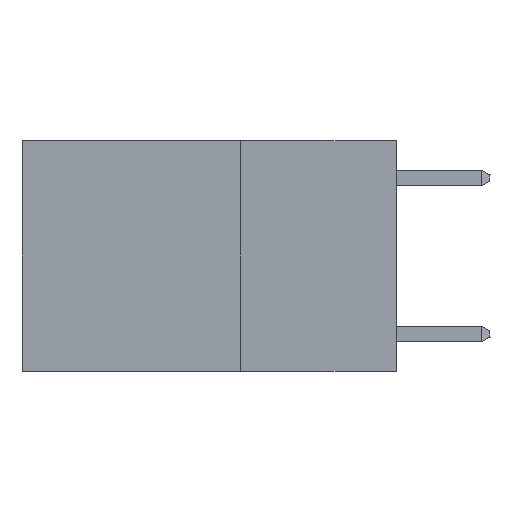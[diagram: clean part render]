
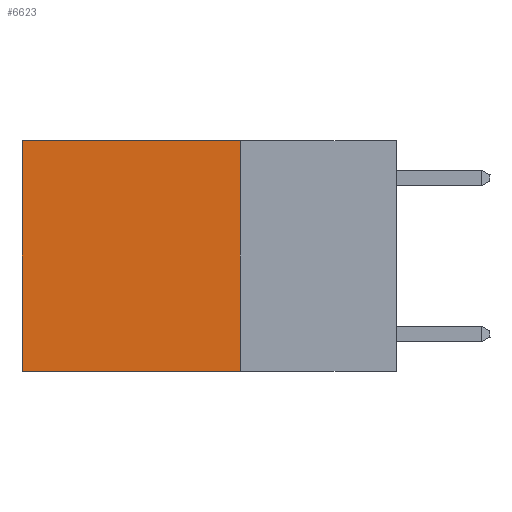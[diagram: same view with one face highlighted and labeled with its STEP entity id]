
A CAD part, left-side view. The second image highlights one B-rep face of the part: STEP entity #6623.
In plain terms, the highlighted planar face has unit normal (-1, 0, 0).
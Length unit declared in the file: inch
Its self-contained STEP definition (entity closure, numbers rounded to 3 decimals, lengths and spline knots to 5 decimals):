
#453 = DIRECTION ( 'NONE',  ( 0., 0., -1. ) ) ;
#927 = EDGE_CURVE ( 'NONE', #4985, #3669, #19596, .T. ) ;
#1441 = LINE ( 'NONE', #14572, #18120 ) ;
#1977 = DIRECTION ( 'NONE',  ( 1., 0., 0. ) ) ;
#2033 = VECTOR ( 'NONE', #16853, 39.37008 ) ;
#2564 = ORIENTED_EDGE ( 'NONE', *, *, #7682, .F. ) ;
#3111 = ORIENTED_EDGE ( 'NONE', *, *, #13722, .F. ) ;
#3427 = EDGE_CURVE ( 'NONE', #3669, #4377, #1441, .T. ) ;
#3669 = VERTEX_POINT ( 'NONE', #17520 ) ;
#4377 = VERTEX_POINT ( 'NONE', #20961 ) ;
#4654 = DIRECTION ( 'NONE',  ( 0., 0., -1. ) ) ;
#4985 = VERTEX_POINT ( 'NONE', #11035 ) ;
#6358 = DIRECTION ( 'NONE',  ( 0., 1., 0. ) ) ;
#6518 = LINE ( 'NONE', #18620, #2033 ) ;
#6623 = ADVANCED_FACE ( 'NONE', ( #8608 ), #10572, .F. ) ;
#6961 = LINE ( 'NONE', #18745, #13705 ) ;
#7682 = EDGE_CURVE ( 'NONE', #4985, #17642, #6961, .T. ) ;
#8608 = FACE_OUTER_BOUND ( 'NONE', #10361, .T. ) ;
#9631 = ORIENTED_EDGE ( 'NONE', *, *, #927, .T. ) ;
#10097 = AXIS2_PLACEMENT_3D ( 'NONE', #17288, #1977, #13884 ) ;
#10361 = EDGE_LOOP ( 'NONE', ( #10643, #3111, #2564, #9631 ) ) ;
#10572 = PLANE ( 'NONE',  #10097 ) ;
#10643 = ORIENTED_EDGE ( 'NONE', *, *, #3427, .T. ) ;
#11035 = CARTESIAN_POINT ( 'NONE',  ( 0.2625, 0.25, 0. ) ) ;
#12118 = CARTESIAN_POINT ( 'NONE',  ( 0.2625, 0.25, -0.37 ) ) ;
#13705 = VECTOR ( 'NONE', #453, 39.37008 ) ;
#13722 = EDGE_CURVE ( 'NONE', #17642, #4377, #6518, .T. ) ;
#13884 = DIRECTION ( 'NONE',  ( 0., 0., -1. ) ) ;
#14572 = CARTESIAN_POINT ( 'NONE',  ( 0.2625, 0.6, 0. ) ) ;
#14734 = CARTESIAN_POINT ( 'NONE',  ( 0.2625, 0.25, 0. ) ) ;
#15001 = VECTOR ( 'NONE', #6358, 39.37008 ) ;
#16853 = DIRECTION ( 'NONE',  ( 0., 1., 0. ) ) ;
#17288 = CARTESIAN_POINT ( 'NONE',  ( 0.2625, 0.25, 0. ) ) ;
#17520 = CARTESIAN_POINT ( 'NONE',  ( 0.2625, 0.6, 0. ) ) ;
#17642 = VERTEX_POINT ( 'NONE', #12118 ) ;
#18120 = VECTOR ( 'NONE', #4654, 39.37008 ) ;
#18620 = CARTESIAN_POINT ( 'NONE',  ( 0.2625, 0.25, -0.37 ) ) ;
#18745 = CARTESIAN_POINT ( 'NONE',  ( 0.2625, 0.25, 0. ) ) ;
#19596 = LINE ( 'NONE', #14734, #15001 ) ;
#20961 = CARTESIAN_POINT ( 'NONE',  ( 0.2625, 0.6, -0.37 ) ) ;
